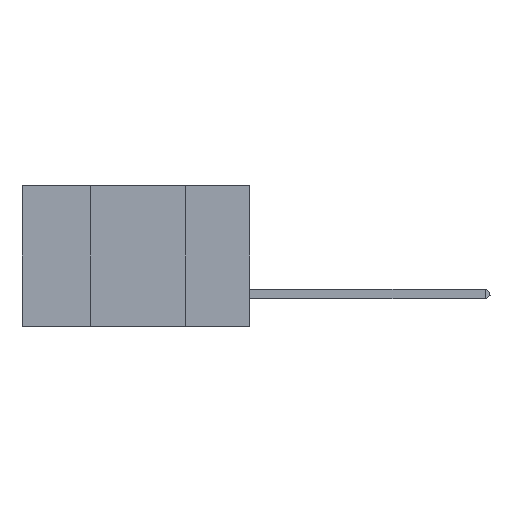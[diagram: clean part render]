
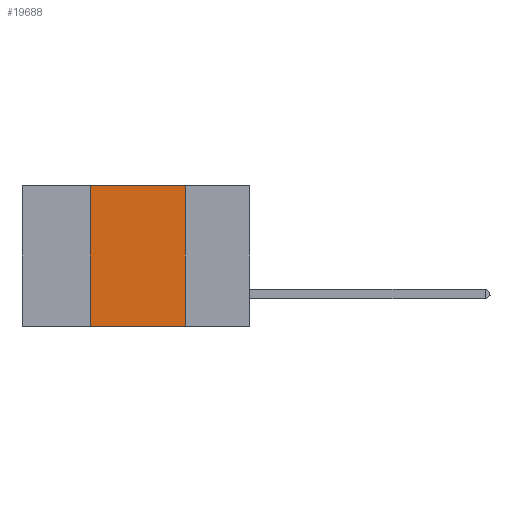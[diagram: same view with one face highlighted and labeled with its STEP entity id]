
A CAD part, left-side view. The second image highlights one B-rep face of the part: STEP entity #19688.
In plain terms, the highlighted planar face has unit normal (-1, 0, 0).
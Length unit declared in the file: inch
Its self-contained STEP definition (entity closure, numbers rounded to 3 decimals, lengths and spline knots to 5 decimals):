
#419 = DIRECTION ( 'NONE',  ( 0., 0., 1. ) ) ;
#494 = VECTOR ( 'NONE', #20448, 39.37008 ) ;
#791 = EDGE_LOOP ( 'NONE', ( #11597, #16300, #18157, #7833 ) ) ;
#1071 = CARTESIAN_POINT ( 'NONE',  ( 0., 0.42, 0. ) ) ;
#1856 = CARTESIAN_POINT ( 'NONE',  ( 0., 0.6, 0. ) ) ;
#1884 = VERTEX_POINT ( 'NONE', #2666 ) ;
#1917 = PLANE ( 'NONE',  #21626 ) ;
#2666 = CARTESIAN_POINT ( 'NONE',  ( 0., 0.42, -0.37 ) ) ;
#2903 = CARTESIAN_POINT ( 'NONE',  ( 0., 0.17, 0. ) ) ;
#3068 = VERTEX_POINT ( 'NONE', #2903 ) ;
#6071 = CARTESIAN_POINT ( 'NONE',  ( 0., 0.17, 0. ) ) ;
#7366 = CARTESIAN_POINT ( 'NONE',  ( 0., 0.17, -0.37 ) ) ;
#7833 = ORIENTED_EDGE ( 'NONE', *, *, #10720, .T. ) ;
#7894 = CARTESIAN_POINT ( 'NONE',  ( 0., 0.6, -0.37 ) ) ;
#7902 = DIRECTION ( 'NONE',  ( 0., 0., -1. ) ) ;
#8185 = FACE_OUTER_BOUND ( 'NONE', #791, .T. ) ;
#8981 = VECTOR ( 'NONE', #13169, 39.37008 ) ;
#9075 = EDGE_CURVE ( 'NONE', #1884, #10887, #15653, .T. ) ;
#9457 = LINE ( 'NONE', #6071, #12607 ) ;
#9834 = VECTOR ( 'NONE', #419, 39.37008 ) ;
#10720 = EDGE_CURVE ( 'NONE', #1884, #16768, #21131, .T. ) ;
#10887 = VERTEX_POINT ( 'NONE', #1071 ) ;
#11081 = EDGE_CURVE ( 'NONE', #10887, #3068, #17668, .T. ) ;
#11597 = ORIENTED_EDGE ( 'NONE', *, *, #17420, .F. ) ;
#12607 = VECTOR ( 'NONE', #7902, 39.37008 ) ;
#13169 = DIRECTION ( 'NONE',  ( 0., -1., 0. ) ) ;
#13731 = DIRECTION ( 'NONE',  ( 1., 0., 0. ) ) ;
#15653 = LINE ( 'NONE', #20950, #9834 ) ;
#16300 = ORIENTED_EDGE ( 'NONE', *, *, #11081, .F. ) ;
#16768 = VERTEX_POINT ( 'NONE', #7366 ) ;
#17420 = EDGE_CURVE ( 'NONE', #3068, #16768, #9457, .T. ) ;
#17668 = LINE ( 'NONE', #1856, #494 ) ;
#18157 = ORIENTED_EDGE ( 'NONE', *, *, #9075, .F. ) ;
#18816 = CARTESIAN_POINT ( 'NONE',  ( 0., 0.6, 0. ) ) ;
#19688 = ADVANCED_FACE ( 'NONE', ( #8185 ), #1917, .F. ) ;
#20448 = DIRECTION ( 'NONE',  ( 0., -1., 0. ) ) ;
#20510 = DIRECTION ( 'NONE',  ( 0., 0., -1. ) ) ;
#20950 = CARTESIAN_POINT ( 'NONE',  ( 0., 0.42, 0. ) ) ;
#21131 = LINE ( 'NONE', #7894, #8981 ) ;
#21626 = AXIS2_PLACEMENT_3D ( 'NONE', #18816, #13731, #20510 ) ;
